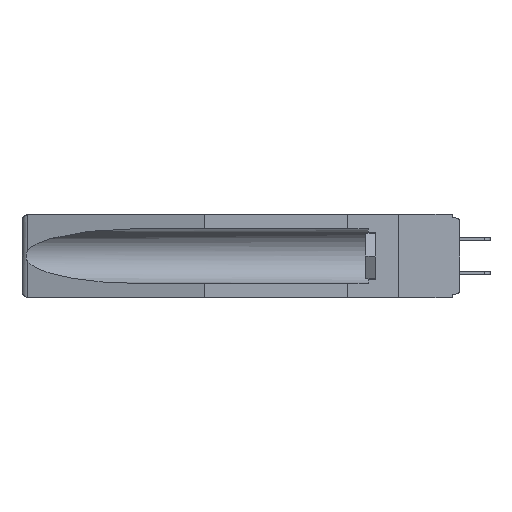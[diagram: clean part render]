
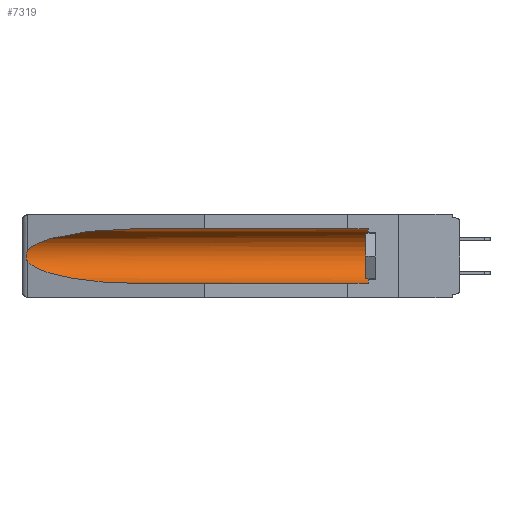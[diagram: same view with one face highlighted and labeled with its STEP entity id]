
A CAD part, left-side view. The second image highlights one B-rep face of the part: STEP entity #7319.
In plain terms, the highlighted cylindrical face has radius 2.857 mm (diameter 5.715 mm), a partial arc.
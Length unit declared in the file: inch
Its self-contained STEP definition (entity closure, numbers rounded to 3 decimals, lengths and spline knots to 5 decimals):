
#161 = CARTESIAN_POINT ( 'NONE',  ( 0.25451, 1.48313, -0.09465 ) ) ;
#738 = LINE ( 'NONE', #19674, #10260 ) ;
#920 = CARTESIAN_POINT ( 'NONE',  ( 0.2675, 1.53308, -0.17534 ) ) ;
#1834 = VECTOR ( 'NONE', #10442, 39.37008 ) ;
#1944 = CARTESIAN_POINT ( 'NONE',  ( 0.155, 1.07973, -0.059 ) ) ;
#2049 = CARTESIAN_POINT ( 'NONE',  ( 0.26537, 1.52718, -0.19328 ) ) ;
#2430 = CARTESIAN_POINT ( 'NONE',  ( 0.155, 1.07973, -0.284 ) ) ;
#2562 = ORIENTED_EDGE ( 'NONE', *, *, #17303, .T. ) ;
#2627 = CARTESIAN_POINT ( 'NONE',  ( 0.26597, 1.5296, -0.19026 ) ) ;
#2782 = CARTESIAN_POINT ( 'NONE',  ( 0.155, 0.126, -0.059 ) ) ;
#2831 = DIRECTION ( 'NONE',  ( 0., 1., 0. ) ) ;
#3053 = DIRECTION ( 'NONE',  ( 0., -1., 0. ) ) ;
#4566 = CARTESIAN_POINT ( 'NONE',  ( 0.155, -0.30754, -0.1715 ) ) ;
#4791 = CARTESIAN_POINT ( 'NONE',  ( 0.155, 0.126, -0.1715 ) ) ;
#5266 =( BOUNDED_CURVE ( )  B_SPLINE_CURVE ( 3, ( #19270, #6165, #9509, #19699 ),
 .UNSPECIFIED., .F., .F. ) 
 B_SPLINE_CURVE_WITH_KNOTS ( ( 4, 4 ),
 ( 0.1948, 1.5708 ),
 .UNSPECIFIED. ) 
 CURVE ( )  GEOMETRIC_REPRESENTATION_ITEM ( )  RATIONAL_B_SPLINE_CURVE ( ( 1., 0.848, 0.848, 1. ) ) 
 REPRESENTATION_ITEM ( '' )  );
#5553 = CARTESIAN_POINT ( 'NONE',  ( 0.155, 0.126, -0.284 ) ) ;
#5939 = VERTEX_POINT ( 'NONE', #1944 ) ;
#6165 = CARTESIAN_POINT ( 'NONE',  ( 0.25451, 1.48313, -0.24835 ) ) ;
#7319 = ADVANCED_FACE ( 'NONE', ( #20221 ), #11735, .F. ) ;
#7589 =( BOUNDED_CURVE ( )  B_SPLINE_CURVE ( 3, ( #14865, #16705, #161, #11899 ),
 .UNSPECIFIED., .F., .F. ) 
 B_SPLINE_CURVE_WITH_KNOTS ( ( 4, 4 ),
 ( 4.71239, 6.08839 ),
 .UNSPECIFIED. ) 
 CURVE ( )  GEOMETRIC_REPRESENTATION_ITEM ( )  RATIONAL_B_SPLINE_CURVE ( ( 1., 0.848, 0.848, 1. ) ) 
 REPRESENTATION_ITEM ( '' )  );
#8258 = AXIS2_PLACEMENT_3D ( 'NONE', #4566, #18041, #13004 ) ;
#9194 = EDGE_CURVE ( 'NONE', #20465, #9900, #5266, .T. ) ;
#9420 = CARTESIAN_POINT ( 'NONE',  ( 0.2673, 1.53269, -0.17917 ) ) ;
#9509 = CARTESIAN_POINT ( 'NONE',  ( 0.21114, 1.30732, -0.284 ) ) ;
#9688 = EDGE_LOOP ( 'NONE', ( #2562, #17196, #20086, #21705, #10142, #9977 ) ) ;
#9747 = VERTEX_POINT ( 'NONE', #5553 ) ;
#9900 = VERTEX_POINT ( 'NONE', #2430 ) ;
#9977 = ORIENTED_EDGE ( 'NONE', *, *, #12235, .T. ) ;
#10003 = LINE ( 'NONE', #15628, #1834 ) ;
#10142 = ORIENTED_EDGE ( 'NONE', *, *, #15278, .T. ) ;
#10260 = VECTOR ( 'NONE', #2831, 39.37008 ) ;
#10442 = DIRECTION ( 'NONE',  ( 0., 1., 0. ) ) ;
#10500 = EDGE_CURVE ( 'NONE', #18325, #20465, #19371, .T. ) ;
#11035 = CARTESIAN_POINT ( 'NONE',  ( 0.2675, 1.53308, -0.16763 ) ) ;
#11651 = AXIS2_PLACEMENT_3D ( 'NONE', #4791, #3053, #18208 ) ;
#11735 = CYLINDRICAL_SURFACE ( 'NONE', #8258, 0.1125 ) ;
#11899 = CARTESIAN_POINT ( 'NONE',  ( 0.26537, 1.52718, -0.14972 ) ) ;
#12235 = EDGE_CURVE ( 'NONE', #18220, #5939, #10003, .T. ) ;
#12737 = CARTESIAN_POINT ( 'NONE',  ( 0.26655, 1.53094, -0.18657 ) ) ;
#13004 = DIRECTION ( 'NONE',  ( 0., 0., 1. ) ) ;
#14865 = CARTESIAN_POINT ( 'NONE',  ( 0.155, 1.07973, -0.059 ) ) ;
#15278 = EDGE_CURVE ( 'NONE', #9747, #18220, #18055, .T. ) ;
#15628 = CARTESIAN_POINT ( 'NONE',  ( 0.155, -0.30754, -0.059 ) ) ;
#16281 = CARTESIAN_POINT ( 'NONE',  ( 0.26597, 1.52961, -0.15275 ) ) ;
#16705 = CARTESIAN_POINT ( 'NONE',  ( 0.21114, 1.30732, -0.059 ) ) ;
#17140 = EDGE_CURVE ( 'NONE', #9747, #9900, #738, .T. ) ;
#17196 = ORIENTED_EDGE ( 'NONE', *, *, #10500, .T. ) ;
#17303 = EDGE_CURVE ( 'NONE', #5939, #18325, #7589, .T. ) ;
#18041 = DIRECTION ( 'NONE',  ( 0., 1., 0. ) ) ;
#18055 = CIRCLE ( 'NONE', #11651, 0.1125 ) ;
#18058 = CARTESIAN_POINT ( 'NONE',  ( 0.26537, 1.52718, -0.14972 ) ) ;
#18208 = DIRECTION ( 'NONE',  ( 0., 0., 1. ) ) ;
#18220 = VERTEX_POINT ( 'NONE', #2782 ) ;
#18297 = CARTESIAN_POINT ( 'NONE',  ( 0.26537, 1.52718, -0.14972 ) ) ;
#18325 = VERTEX_POINT ( 'NONE', #18297 ) ;
#19270 = CARTESIAN_POINT ( 'NONE',  ( 0.26537, 1.52718, -0.19328 ) ) ;
#19371 = B_SPLINE_CURVE_WITH_KNOTS ( 'NONE', 3,
 ( #18058, #16281, #19551, #21167, #11035, #920, #9420, #12737, #2627, #19970 ),
 .UNSPECIFIED., .F., .F.,
 ( 4, 2, 2, 2, 4 ),
 ( 0., 0.00029, 0.00058, 0.00087, 0.00117 ),
 .UNSPECIFIED. ) ;
#19551 = CARTESIAN_POINT ( 'NONE',  ( 0.26654, 1.53092, -0.15636 ) ) ;
#19674 = CARTESIAN_POINT ( 'NONE',  ( 0.155, -0.30754, -0.284 ) ) ;
#19699 = CARTESIAN_POINT ( 'NONE',  ( 0.155, 1.07973, -0.284 ) ) ;
#19970 = CARTESIAN_POINT ( 'NONE',  ( 0.26537, 1.52718, -0.19328 ) ) ;
#20086 = ORIENTED_EDGE ( 'NONE', *, *, #9194, .T. ) ;
#20221 = FACE_OUTER_BOUND ( 'NONE', #9688, .T. ) ;
#20465 = VERTEX_POINT ( 'NONE', #2049 ) ;
#21167 = CARTESIAN_POINT ( 'NONE',  ( 0.2673, 1.5327, -0.16383 ) ) ;
#21705 = ORIENTED_EDGE ( 'NONE', *, *, #17140, .F. ) ;
